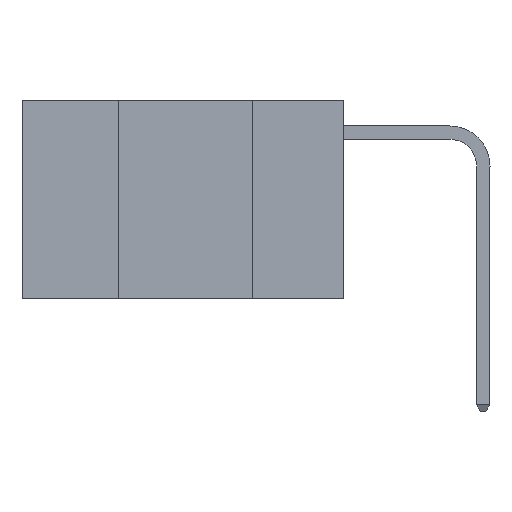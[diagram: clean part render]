
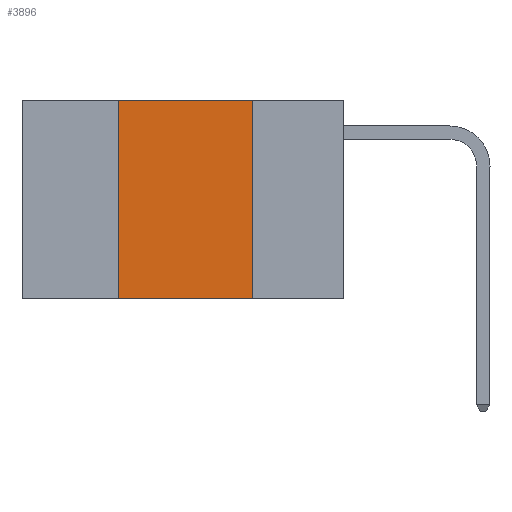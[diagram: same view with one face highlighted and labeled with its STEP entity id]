
A CAD part, left-side view. The second image highlights one B-rep face of the part: STEP entity #3896.
In plain terms, the highlighted planar face has unit normal (-1, 0, 0).
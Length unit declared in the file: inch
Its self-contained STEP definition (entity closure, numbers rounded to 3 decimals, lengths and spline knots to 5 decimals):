
#672 = VERTEX_POINT ( 'NONE', #11273 ) ;
#1615 = VERTEX_POINT ( 'NONE', #11290 ) ;
#2239 = VECTOR ( 'NONE', #6166, 39.37008 ) ;
#2256 = VERTEX_POINT ( 'NONE', #14327 ) ;
#2662 = LINE ( 'NONE', #6912, #8877 ) ;
#2718 = ORIENTED_EDGE ( 'NONE', *, *, #5871, .T. ) ;
#3896 = ADVANCED_FACE ( 'NONE', ( #10045 ), #7672, .F. ) ;
#4016 = CARTESIAN_POINT ( 'NONE',  ( 0., 0.6, 0. ) ) ;
#5242 = DIRECTION ( 'NONE',  ( 0., 0., -1. ) ) ;
#5428 = EDGE_CURVE ( 'NONE', #7352, #1615, #5988, .T. ) ;
#5652 = ORIENTED_EDGE ( 'NONE', *, *, #15705, .F. ) ;
#5871 = EDGE_CURVE ( 'NONE', #672, #1615, #15456, .T. ) ;
#5988 = LINE ( 'NONE', #9027, #15469 ) ;
#6089 = EDGE_LOOP ( 'NONE', ( #8548, #5652, #15537, #2718 ) ) ;
#6166 = DIRECTION ( 'NONE',  ( 0., -1., 0. ) ) ;
#6601 = EDGE_CURVE ( 'NONE', #672, #2256, #11058, .T. ) ;
#6912 = CARTESIAN_POINT ( 'NONE',  ( 0., 0.6, 0. ) ) ;
#7299 = VECTOR ( 'NONE', #7740, 39.37008 ) ;
#7352 = VERTEX_POINT ( 'NONE', #9200 ) ;
#7672 = PLANE ( 'NONE',  #9169 ) ;
#7740 = DIRECTION ( 'NONE',  ( 0., 0., 1. ) ) ;
#8548 = ORIENTED_EDGE ( 'NONE', *, *, #5428, .F. ) ;
#8877 = VECTOR ( 'NONE', #13189, 39.37008 ) ;
#8992 = CARTESIAN_POINT ( 'NONE',  ( 0., 0.42, 0. ) ) ;
#9027 = CARTESIAN_POINT ( 'NONE',  ( 0., 0.17, 0. ) ) ;
#9169 = AXIS2_PLACEMENT_3D ( 'NONE', #4016, #12765, #5242 ) ;
#9200 = CARTESIAN_POINT ( 'NONE',  ( 0., 0.17, 0. ) ) ;
#10045 = FACE_OUTER_BOUND ( 'NONE', #6089, .T. ) ;
#11058 = LINE ( 'NONE', #8992, #7299 ) ;
#11273 = CARTESIAN_POINT ( 'NONE',  ( 0., 0.42, -0.37 ) ) ;
#11290 = CARTESIAN_POINT ( 'NONE',  ( 0., 0.17, -0.37 ) ) ;
#11575 = DIRECTION ( 'NONE',  ( 0., 0., -1. ) ) ;
#12765 = DIRECTION ( 'NONE',  ( 1., 0., 0. ) ) ;
#13189 = DIRECTION ( 'NONE',  ( 0., -1., 0. ) ) ;
#14327 = CARTESIAN_POINT ( 'NONE',  ( 0., 0.42, 0. ) ) ;
#14839 = CARTESIAN_POINT ( 'NONE',  ( 0., 0.6, -0.37 ) ) ;
#15456 = LINE ( 'NONE', #14839, #2239 ) ;
#15469 = VECTOR ( 'NONE', #11575, 39.37008 ) ;
#15537 = ORIENTED_EDGE ( 'NONE', *, *, #6601, .F. ) ;
#15705 = EDGE_CURVE ( 'NONE', #2256, #7352, #2662, .T. ) ;
